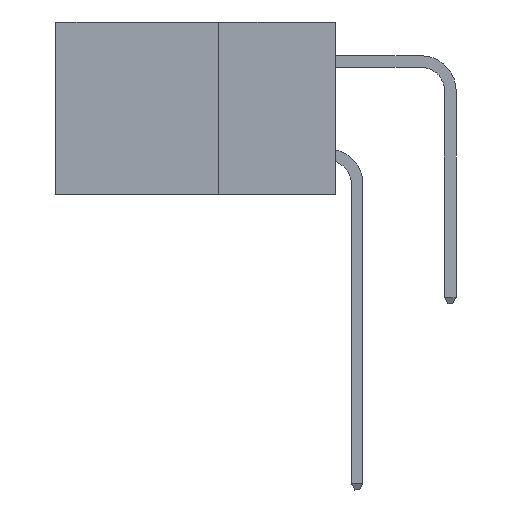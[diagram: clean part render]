
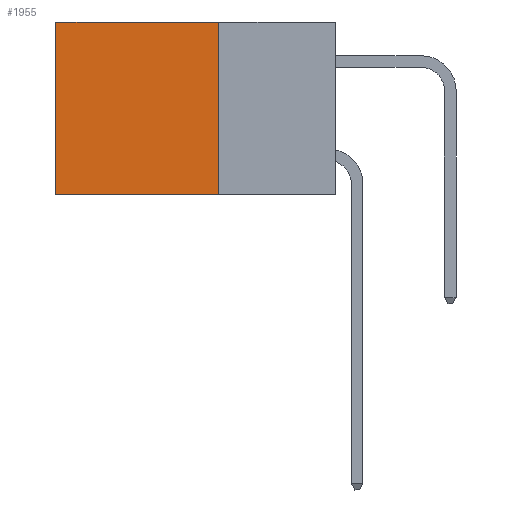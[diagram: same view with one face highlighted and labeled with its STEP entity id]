
A CAD part, left-side view. The second image highlights one B-rep face of the part: STEP entity #1955.
In plain terms, the highlighted planar face has unit normal (-1, 0, 0).
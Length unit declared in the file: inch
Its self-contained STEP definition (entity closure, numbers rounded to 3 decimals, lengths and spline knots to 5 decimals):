
#1955 = ADVANCED_FACE ( 'NONE', ( #5502 ), #3445, .F. ) ;
#2003 = DIRECTION ( 'NONE',  ( 0., 0., -1. ) ) ;
#2121 = ORIENTED_EDGE ( 'NONE', *, *, #8907, .T. ) ;
#2485 = ORIENTED_EDGE ( 'NONE', *, *, #7826, .F. ) ;
#2550 = DIRECTION ( 'NONE',  ( 0., 0., -1. ) ) ;
#3177 = CARTESIAN_POINT ( 'NONE',  ( 0.2875, 0.25, 0. ) ) ;
#3445 = PLANE ( 'NONE',  #10150 ) ;
#3591 = DIRECTION ( 'NONE',  ( 0., 1., 0. ) ) ;
#3673 = LINE ( 'NONE', #6587, #11224 ) ;
#3941 = VECTOR ( 'NONE', #3591, 39.37008 ) ;
#3943 = VECTOR ( 'NONE', #11520, 39.37008 ) ;
#4116 = LINE ( 'NONE', #8378, #3941 ) ;
#5317 = DIRECTION ( 'NONE',  ( 0., 1., 0. ) ) ;
#5502 = FACE_OUTER_BOUND ( 'NONE', #14448, .T. ) ;
#5951 = VERTEX_POINT ( 'NONE', #10167 ) ;
#6324 = VECTOR ( 'NONE', #2550, 39.37008 ) ;
#6587 = CARTESIAN_POINT ( 'NONE',  ( 0.2875, 0.25, 0. ) ) ;
#7826 = EDGE_CURVE ( 'NONE', #8838, #11547, #4116, .T. ) ;
#8378 = CARTESIAN_POINT ( 'NONE',  ( 0.2875, 0.25, -0.37 ) ) ;
#8838 = VERTEX_POINT ( 'NONE', #9542 ) ;
#8907 = EDGE_CURVE ( 'NONE', #9766, #5951, #3673, .T. ) ;
#9542 = CARTESIAN_POINT ( 'NONE',  ( 0.2875, 0.25, -0.37 ) ) ;
#9766 = VERTEX_POINT ( 'NONE', #3177 ) ;
#10150 = AXIS2_PLACEMENT_3D ( 'NONE', #11803, #15348, #2003 ) ;
#10167 = CARTESIAN_POINT ( 'NONE',  ( 0.2875, 0.6, 0. ) ) ;
#10830 = EDGE_CURVE ( 'NONE', #5951, #11547, #13626, .T. ) ;
#11221 = CARTESIAN_POINT ( 'NONE',  ( 0.2875, 0.6, 0. ) ) ;
#11224 = VECTOR ( 'NONE', #5317, 39.37008 ) ;
#11451 = ORIENTED_EDGE ( 'NONE', *, *, #13918, .F. ) ;
#11520 = DIRECTION ( 'NONE',  ( 0., 0., -1. ) ) ;
#11547 = VERTEX_POINT ( 'NONE', #14340 ) ;
#11803 = CARTESIAN_POINT ( 'NONE',  ( 0.2875, 0.25, 0. ) ) ;
#13343 = LINE ( 'NONE', #14693, #6324 ) ;
#13626 = LINE ( 'NONE', #11221, #3943 ) ;
#13918 = EDGE_CURVE ( 'NONE', #9766, #8838, #13343, .T. ) ;
#14340 = CARTESIAN_POINT ( 'NONE',  ( 0.2875, 0.6, -0.37 ) ) ;
#14448 = EDGE_LOOP ( 'NONE', ( #15630, #2485, #11451, #2121 ) ) ;
#14693 = CARTESIAN_POINT ( 'NONE',  ( 0.2875, 0.25, 0. ) ) ;
#15348 = DIRECTION ( 'NONE',  ( 1., 0., 0. ) ) ;
#15630 = ORIENTED_EDGE ( 'NONE', *, *, #10830, .T. ) ;
